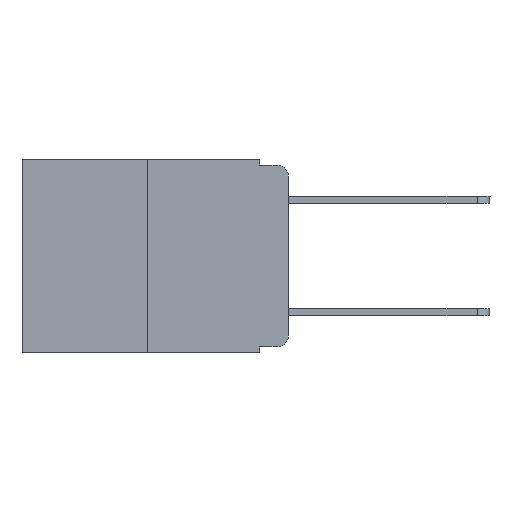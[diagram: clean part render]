
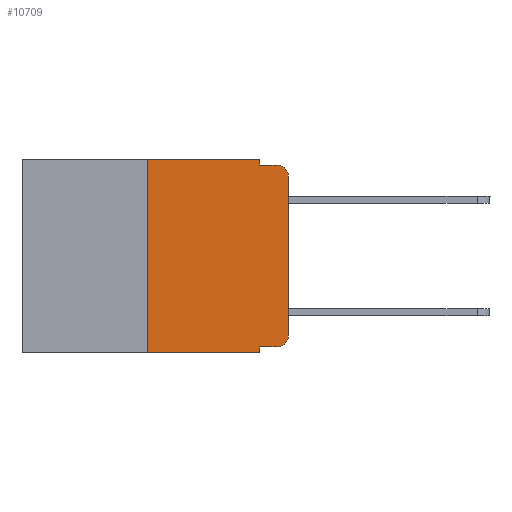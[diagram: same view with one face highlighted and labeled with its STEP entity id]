
A CAD part, left-side view. The second image highlights one B-rep face of the part: STEP entity #10709.
In plain terms, the highlighted planar face has unit normal (-1, 0, 0).
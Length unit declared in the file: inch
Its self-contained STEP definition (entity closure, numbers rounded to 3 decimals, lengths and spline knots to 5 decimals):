
#127 = LINE ( 'NONE', #16463, #14366 ) ;
#278 = EDGE_CURVE ( 'NONE', #19170, #2793, #1738, .T. ) ;
#450 = VERTEX_POINT ( 'NONE', #6777 ) ;
#527 = CARTESIAN_POINT ( 'NONE',  ( 0., 0., 0. ) ) ;
#1431 = CARTESIAN_POINT ( 'NONE',  ( 0., 0.051, 0. ) ) ;
#1588 = VECTOR ( 'NONE', #5170, 39.37008 ) ;
#1600 = ORIENTED_EDGE ( 'NONE', *, *, #11051, .F. ) ;
#1738 = LINE ( 'NONE', #7870, #5812 ) ;
#1914 = ORIENTED_EDGE ( 'NONE', *, *, #9694, .F. ) ;
#2074 = VERTEX_POINT ( 'NONE', #16355 ) ;
#2266 = DIRECTION ( 'NONE',  ( 0., 0., 1. ) ) ;
#2793 = VERTEX_POINT ( 'NONE', #8732 ) ;
#2995 = VERTEX_POINT ( 'NONE', #17360 ) ;
#3412 = PLANE ( 'NONE',  #5629 ) ;
#3515 = FACE_OUTER_BOUND ( 'NONE', #11408, .T. ) ;
#3692 = CARTESIAN_POINT ( 'NONE',  ( 0., 0.473, 0. ) ) ;
#3739 = AXIS2_PLACEMENT_3D ( 'NONE', #8205, #12537, #18628 ) ;
#3776 = VECTOR ( 'NONE', #13019, 39.37008 ) ;
#4109 = CARTESIAN_POINT ( 'NONE',  ( 0., 0.051, 0. ) ) ;
#4762 = ORIENTED_EDGE ( 'NONE', *, *, #15230, .T. ) ;
#4869 = CARTESIAN_POINT ( 'NONE',  ( 0., 0.25, 0. ) ) ;
#4907 = CARTESIAN_POINT ( 'NONE',  ( 0., 0., -0.313 ) ) ;
#5170 = DIRECTION ( 'NONE',  ( 0., 0., 1. ) ) ;
#5288 = ORIENTED_EDGE ( 'NONE', *, *, #10796, .F. ) ;
#5629 = AXIS2_PLACEMENT_3D ( 'NONE', #3692, #6424, #15556 ) ;
#5812 = VECTOR ( 'NONE', #12589, 39.37008 ) ;
#6040 = CARTESIAN_POINT ( 'NONE',  ( 0., 0.25, -0.343 ) ) ;
#6269 = VECTOR ( 'NONE', #2266, 39.37008 ) ;
#6424 = DIRECTION ( 'NONE',  ( 1., 0., 0. ) ) ;
#6518 = LINE ( 'NONE', #17215, #1588 ) ;
#6525 = VECTOR ( 'NONE', #8231, 39.37008 ) ;
#6777 = CARTESIAN_POINT ( 'NONE',  ( 0., 0.02, -0.01 ) ) ;
#7773 = ORIENTED_EDGE ( 'NONE', *, *, #10215, .T. ) ;
#7870 = CARTESIAN_POINT ( 'NONE',  ( 0., 0.473, 0. ) ) ;
#8205 = CARTESIAN_POINT ( 'NONE',  ( 0., 0.02, -0.313 ) ) ;
#8231 = DIRECTION ( 'NONE',  ( 0., -1., 0. ) ) ;
#8280 = VERTEX_POINT ( 'NONE', #9714 ) ;
#8732 = CARTESIAN_POINT ( 'NONE',  ( 0., 0.051, 0. ) ) ;
#8956 = LINE ( 'NONE', #14939, #6525 ) ;
#9066 = VERTEX_POINT ( 'NONE', #6040 ) ;
#9421 = ORIENTED_EDGE ( 'NONE', *, *, #9492, .T. ) ;
#9492 = EDGE_CURVE ( 'NONE', #2074, #8280, #8956, .T. ) ;
#9501 = CARTESIAN_POINT ( 'NONE',  ( 0., 0.473, -0.343 ) ) ;
#9694 = EDGE_CURVE ( 'NONE', #2995, #450, #127, .T. ) ;
#9714 = CARTESIAN_POINT ( 'NONE',  ( 0., 0.02, -0.333 ) ) ;
#9849 = VERTEX_POINT ( 'NONE', #4907 ) ;
#10215 = EDGE_CURVE ( 'NONE', #8280, #9849, #18780, .T. ) ;
#10328 = LINE ( 'NONE', #1431, #11579 ) ;
#10642 = ORIENTED_EDGE ( 'NONE', *, *, #16805, .F. ) ;
#10709 = ADVANCED_FACE ( 'NONE', ( #3515 ), #3412, .F. ) ;
#10787 = CARTESIAN_POINT ( 'NONE',  ( 0., 0.02, -0.03 ) ) ;
#10796 = EDGE_CURVE ( 'NONE', #9066, #19170, #6518, .T. ) ;
#10881 = LINE ( 'NONE', #527, #6269 ) ;
#11024 = VECTOR ( 'NONE', #14391, 39.37008 ) ;
#11051 = EDGE_CURVE ( 'NONE', #2074, #17523, #10328, .T. ) ;
#11294 = CARTESIAN_POINT ( 'NONE',  ( 0., 0.051, -0.343 ) ) ;
#11408 = EDGE_LOOP ( 'NONE', ( #4762, #15893, #1914, #10642, #11813, #5288, #12505, #1600, #9421, #7773 ) ) ;
#11446 = LINE ( 'NONE', #9501, #3776 ) ;
#11579 = VECTOR ( 'NONE', #11897, 39.37008 ) ;
#11731 = EDGE_CURVE ( 'NONE', #9066, #17523, #11446, .T. ) ;
#11813 = ORIENTED_EDGE ( 'NONE', *, *, #278, .F. ) ;
#11897 = DIRECTION ( 'NONE',  ( 0., 0., -1. ) ) ;
#11981 = AXIS2_PLACEMENT_3D ( 'NONE', #10787, #13637, #12270 ) ;
#12270 = DIRECTION ( 'NONE',  ( 0., 0., -1. ) ) ;
#12505 = ORIENTED_EDGE ( 'NONE', *, *, #11731, .T. ) ;
#12537 = DIRECTION ( 'NONE',  ( -1., 0., 0. ) ) ;
#12589 = DIRECTION ( 'NONE',  ( 0., -1., 0. ) ) ;
#13019 = DIRECTION ( 'NONE',  ( 0., -1., 0. ) ) ;
#13637 = DIRECTION ( 'NONE',  ( -1., 0., 0. ) ) ;
#14366 = VECTOR ( 'NONE', #16171, 39.37008 ) ;
#14391 = DIRECTION ( 'NONE',  ( 0., 0., -1. ) ) ;
#14482 = CIRCLE ( 'NONE', #11981, 0.02 ) ;
#14773 = VERTEX_POINT ( 'NONE', #18374 ) ;
#14939 = CARTESIAN_POINT ( 'NONE',  ( 0., 0.051, -0.333 ) ) ;
#15230 = EDGE_CURVE ( 'NONE', #9849, #14773, #10881, .T. ) ;
#15556 = DIRECTION ( 'NONE',  ( 0., 0., -1. ) ) ;
#15893 = ORIENTED_EDGE ( 'NONE', *, *, #17796, .T. ) ;
#16171 = DIRECTION ( 'NONE',  ( 0., -1., 0. ) ) ;
#16355 = CARTESIAN_POINT ( 'NONE',  ( 0., 0.051, -0.333 ) ) ;
#16463 = CARTESIAN_POINT ( 'NONE',  ( 0., 0.051, -0.01 ) ) ;
#16805 = EDGE_CURVE ( 'NONE', #2793, #2995, #18932, .T. ) ;
#17215 = CARTESIAN_POINT ( 'NONE',  ( 0., 0.25, 0. ) ) ;
#17360 = CARTESIAN_POINT ( 'NONE',  ( 0., 0.051, -0.01 ) ) ;
#17523 = VERTEX_POINT ( 'NONE', #11294 ) ;
#17796 = EDGE_CURVE ( 'NONE', #14773, #450, #14482, .T. ) ;
#18374 = CARTESIAN_POINT ( 'NONE',  ( 0., 0., -0.03 ) ) ;
#18628 = DIRECTION ( 'NONE',  ( 0., 0., -1. ) ) ;
#18780 = CIRCLE ( 'NONE', #3739, 0.02 ) ;
#18932 = LINE ( 'NONE', #4109, #11024 ) ;
#19170 = VERTEX_POINT ( 'NONE', #4869 ) ;
